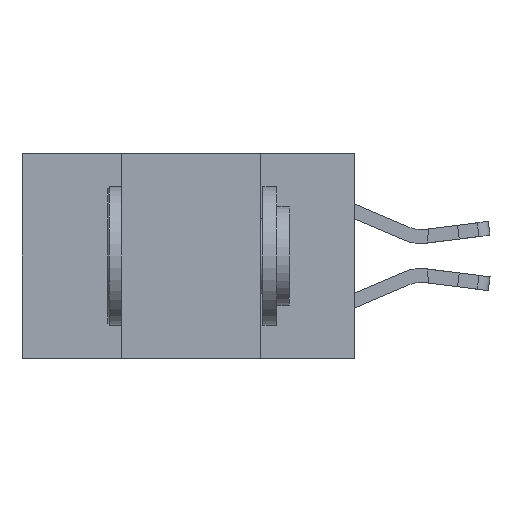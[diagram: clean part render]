
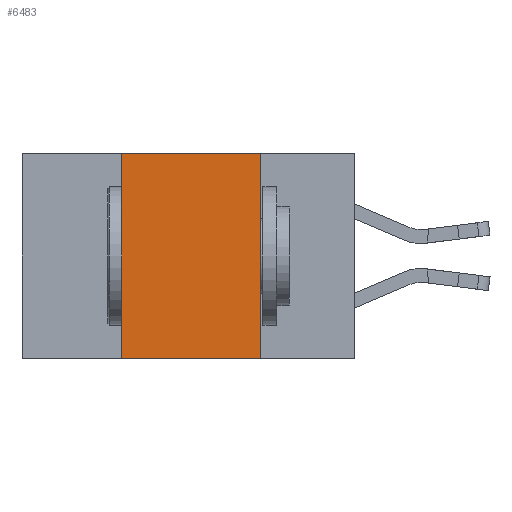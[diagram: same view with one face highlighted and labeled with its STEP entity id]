
A CAD part, left-side view. The second image highlights one B-rep face of the part: STEP entity #6483.
In plain terms, the highlighted planar face has unit normal (-1, 0, 0).
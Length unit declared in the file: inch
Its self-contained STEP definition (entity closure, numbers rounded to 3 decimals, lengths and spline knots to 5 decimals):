
#1165 = AXIS2_PLACEMENT_3D ( 'NONE', #12119, #6372, #7432 ) ;
#2000 = LINE ( 'NONE', #12158, #4825 ) ;
#2449 = CARTESIAN_POINT ( 'NONE',  ( 0., 0.17, 0. ) ) ;
#2673 = VERTEX_POINT ( 'NONE', #3695 ) ;
#3138 = EDGE_LOOP ( 'NONE', ( #7502, #11908, #4442, #3299 ) ) ;
#3178 = LINE ( 'NONE', #7456, #4993 ) ;
#3299 = ORIENTED_EDGE ( 'NONE', *, *, #4441, .T. ) ;
#3695 = CARTESIAN_POINT ( 'NONE',  ( 0., 0.42, -0.37 ) ) ;
#4151 = CARTESIAN_POINT ( 'NONE',  ( 0., 0.17, 0. ) ) ;
#4250 = LINE ( 'NONE', #2449, #9330 ) ;
#4441 = EDGE_CURVE ( 'NONE', #2673, #10470, #3178, .T. ) ;
#4442 = ORIENTED_EDGE ( 'NONE', *, *, #11002, .F. ) ;
#4825 = VECTOR ( 'NONE', #8373, 39.37008 ) ;
#4939 = VERTEX_POINT ( 'NONE', #8392 ) ;
#4993 = VECTOR ( 'NONE', #6559, 39.37008 ) ;
#5605 = LINE ( 'NONE', #8557, #8458 ) ;
#6155 = FACE_OUTER_BOUND ( 'NONE', #3138, .T. ) ;
#6353 = CARTESIAN_POINT ( 'NONE',  ( 0., 0.17, -0.37 ) ) ;
#6372 = DIRECTION ( 'NONE',  ( 1., 0., 0. ) ) ;
#6483 = ADVANCED_FACE ( 'NONE', ( #6155 ), #10963, .F. ) ;
#6559 = DIRECTION ( 'NONE',  ( 0., -1., 0. ) ) ;
#7038 = VERTEX_POINT ( 'NONE', #4151 ) ;
#7432 = DIRECTION ( 'NONE',  ( 0., 0., -1. ) ) ;
#7456 = CARTESIAN_POINT ( 'NONE',  ( 0., 0.6, -0.37 ) ) ;
#7502 = ORIENTED_EDGE ( 'NONE', *, *, #10944, .F. ) ;
#8373 = DIRECTION ( 'NONE',  ( 0., -1., 0. ) ) ;
#8392 = CARTESIAN_POINT ( 'NONE',  ( 0., 0.42, 0. ) ) ;
#8458 = VECTOR ( 'NONE', #11264, 39.37008 ) ;
#8557 = CARTESIAN_POINT ( 'NONE',  ( 0., 0.42, 0. ) ) ;
#9330 = VECTOR ( 'NONE', #10131, 39.37008 ) ;
#10131 = DIRECTION ( 'NONE',  ( 0., 0., -1. ) ) ;
#10470 = VERTEX_POINT ( 'NONE', #6353 ) ;
#10944 = EDGE_CURVE ( 'NONE', #7038, #10470, #4250, .T. ) ;
#10963 = PLANE ( 'NONE',  #1165 ) ;
#11002 = EDGE_CURVE ( 'NONE', #2673, #4939, #5605, .T. ) ;
#11264 = DIRECTION ( 'NONE',  ( 0., 0., 1. ) ) ;
#11908 = ORIENTED_EDGE ( 'NONE', *, *, #11948, .F. ) ;
#11948 = EDGE_CURVE ( 'NONE', #4939, #7038, #2000, .T. ) ;
#12119 = CARTESIAN_POINT ( 'NONE',  ( 0., 0.6, 0. ) ) ;
#12158 = CARTESIAN_POINT ( 'NONE',  ( 0., 0.6, 0. ) ) ;
